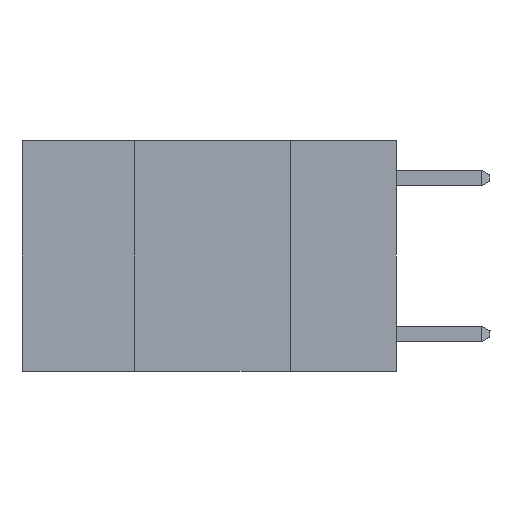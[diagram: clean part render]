
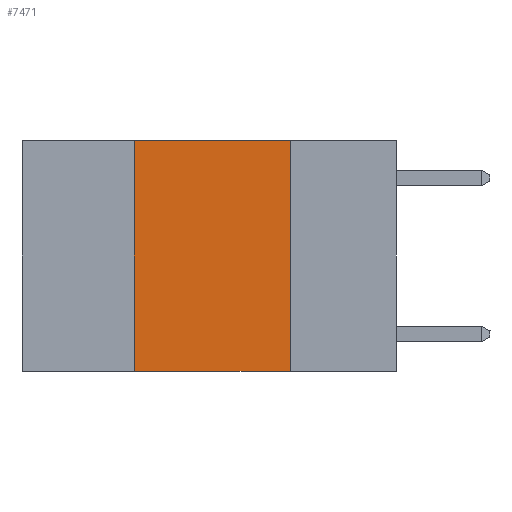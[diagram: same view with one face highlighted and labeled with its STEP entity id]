
A CAD part, left-side view. The second image highlights one B-rep face of the part: STEP entity #7471.
In plain terms, the highlighted planar face has unit normal (-1, 0, 0).
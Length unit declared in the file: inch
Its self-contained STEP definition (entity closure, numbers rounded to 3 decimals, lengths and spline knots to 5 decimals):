
#340 = DIRECTION ( 'NONE',  ( 1., 0., 0. ) ) ;
#764 = DIRECTION ( 'NONE',  ( 0., 0., 1. ) ) ;
#2024 = VECTOR ( 'NONE', #764, 39.37008 ) ;
#2036 = LINE ( 'NONE', #3715, #4306 ) ;
#2509 = LINE ( 'NONE', #8836, #11685 ) ;
#2516 = VERTEX_POINT ( 'NONE', #10776 ) ;
#3242 = DIRECTION ( 'NONE',  ( 0., 0., -1. ) ) ;
#3715 = CARTESIAN_POINT ( 'NONE',  ( 0., 0.6, 0. ) ) ;
#3745 = CARTESIAN_POINT ( 'NONE',  ( 0., 0.6, -0.37 ) ) ;
#4306 = VECTOR ( 'NONE', #10174, 39.37008 ) ;
#5421 = CARTESIAN_POINT ( 'NONE',  ( 0., 0.42, -0.37 ) ) ;
#5776 = CARTESIAN_POINT ( 'NONE',  ( 0., 0.17, -0.37 ) ) ;
#6121 = PLANE ( 'NONE',  #7307 ) ;
#6501 = LINE ( 'NONE', #3745, #11016 ) ;
#7017 = DIRECTION ( 'NONE',  ( 0., 0., -1. ) ) ;
#7239 = VERTEX_POINT ( 'NONE', #5776 ) ;
#7307 = AXIS2_PLACEMENT_3D ( 'NONE', #8797, #340, #7017 ) ;
#7471 = ADVANCED_FACE ( 'NONE', ( #10923 ), #6121, .F. ) ;
#7486 = DIRECTION ( 'NONE',  ( 0., -1., 0. ) ) ;
#7743 = ORIENTED_EDGE ( 'NONE', *, *, #10153, .F. ) ;
#8337 = CARTESIAN_POINT ( 'NONE',  ( 0., 0.42, 0. ) ) ;
#8404 = ORIENTED_EDGE ( 'NONE', *, *, #10866, .F. ) ;
#8797 = CARTESIAN_POINT ( 'NONE',  ( 0., 0.6, 0. ) ) ;
#8836 = CARTESIAN_POINT ( 'NONE',  ( 0., 0.17, 0. ) ) ;
#9283 = ORIENTED_EDGE ( 'NONE', *, *, #10933, .T. ) ;
#9706 = CARTESIAN_POINT ( 'NONE',  ( 0., 0.42, 0. ) ) ;
#9763 = ORIENTED_EDGE ( 'NONE', *, *, #10414, .F. ) ;
#9974 = EDGE_LOOP ( 'NONE', ( #9763, #7743, #8404, #9283 ) ) ;
#10153 = EDGE_CURVE ( 'NONE', #11777, #2516, #2036, .T. ) ;
#10174 = DIRECTION ( 'NONE',  ( 0., -1., 0. ) ) ;
#10414 = EDGE_CURVE ( 'NONE', #2516, #7239, #2509, .T. ) ;
#10702 = VERTEX_POINT ( 'NONE', #5421 ) ;
#10776 = CARTESIAN_POINT ( 'NONE',  ( 0., 0.17, 0. ) ) ;
#10866 = EDGE_CURVE ( 'NONE', #10702, #11777, #11540, .T. ) ;
#10923 = FACE_OUTER_BOUND ( 'NONE', #9974, .T. ) ;
#10933 = EDGE_CURVE ( 'NONE', #10702, #7239, #6501, .T. ) ;
#11016 = VECTOR ( 'NONE', #7486, 39.37008 ) ;
#11540 = LINE ( 'NONE', #8337, #2024 ) ;
#11685 = VECTOR ( 'NONE', #3242, 39.37008 ) ;
#11777 = VERTEX_POINT ( 'NONE', #9706 ) ;
